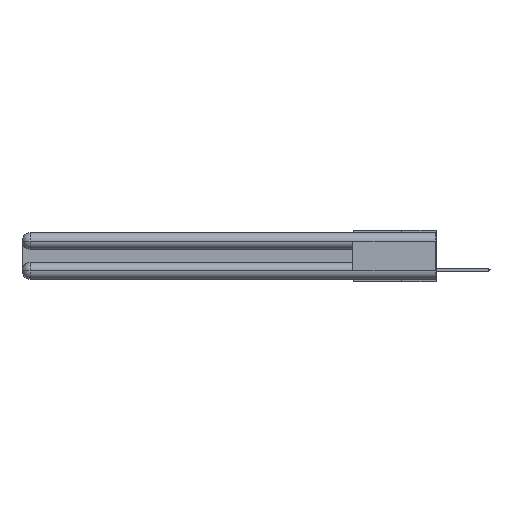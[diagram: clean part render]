
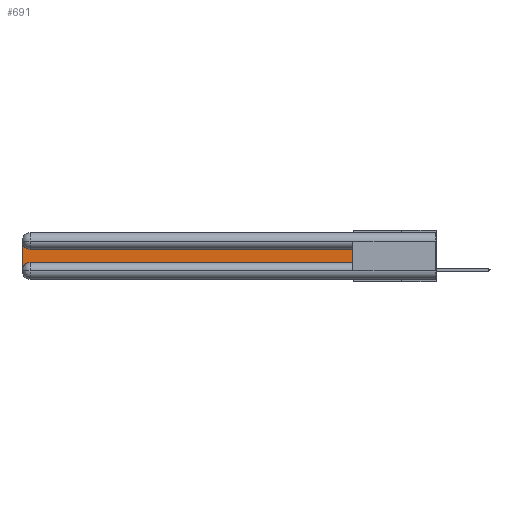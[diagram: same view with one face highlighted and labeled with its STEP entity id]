
A CAD part, left-side view. The second image highlights one B-rep face of the part: STEP entity #691.
In plain terms, the highlighted planar face has unit normal (-1, 0, 0).
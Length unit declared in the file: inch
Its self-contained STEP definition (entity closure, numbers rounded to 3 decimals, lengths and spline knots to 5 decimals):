
#261 = CARTESIAN_POINT ( 'NONE',  ( 0.075, 0.6, -0.2175 ) ) ;
#691 = ADVANCED_FACE ( 'NONE', ( #5377 ), #24101, .F. ) ;
#938 = CARTESIAN_POINT ( 'NONE',  ( 0.075, 0.6, -0.1225 ) ) ;
#1121 = DIRECTION ( 'NONE',  ( 0., 0., 1. ) ) ;
#1133 = CIRCLE ( 'NONE', #24353, 0.06 ) ;
#1188 = DIRECTION ( 'NONE',  ( 1., 0., 0. ) ) ;
#2538 = VERTEX_POINT ( 'NONE', #26113 ) ;
#2850 = DIRECTION ( 'NONE',  ( 1., 0., 0. ) ) ;
#3032 = VECTOR ( 'NONE', #1121, 39.37008 ) ;
#3155 = EDGE_CURVE ( 'NONE', #12133, #13346, #20397, .T. ) ;
#3655 = AXIS2_PLACEMENT_3D ( 'NONE', #5633, #14016, #5889 ) ;
#4423 = AXIS2_PLACEMENT_3D ( 'NONE', #25682, #1188, #17885 ) ;
#4706 = DIRECTION ( 'NONE',  ( 0., 0., -1. ) ) ;
#4826 = CARTESIAN_POINT ( 'NONE',  ( 0.075, 2.94, -0.0625 ) ) ;
#5377 = FACE_OUTER_BOUND ( 'NONE', #7575, .T. ) ;
#5633 = CARTESIAN_POINT ( 'NONE',  ( 0.075, 3., -0.1225 ) ) ;
#5889 = DIRECTION ( 'NONE',  ( 0., 0., -1. ) ) ;
#6248 = VERTEX_POINT ( 'NONE', #18762 ) ;
#6718 = EDGE_CURVE ( 'NONE', #15944, #20426, #1133, .T. ) ;
#7150 = CARTESIAN_POINT ( 'NONE',  ( 0.075, 3., -0.0625 ) ) ;
#7454 = DIRECTION ( 'NONE',  ( 0., 1., 0. ) ) ;
#7575 = EDGE_LOOP ( 'NONE', ( #8621, #14292, #20727, #9318, #16063, #13437 ) ) ;
#8621 = ORIENTED_EDGE ( 'NONE', *, *, #22195, .T. ) ;
#9318 = ORIENTED_EDGE ( 'NONE', *, *, #10266, .T. ) ;
#10266 = EDGE_CURVE ( 'NONE', #2538, #6248, #14144, .T. ) ;
#10718 = CARTESIAN_POINT ( 'NONE',  ( 0.075, 0.6, -0.2175 ) ) ;
#12133 = VERTEX_POINT ( 'NONE', #261 ) ;
#12501 = VECTOR ( 'NONE', #7454, 39.37008 ) ;
#13346 = VERTEX_POINT ( 'NONE', #25940 ) ;
#13437 = ORIENTED_EDGE ( 'NONE', *, *, #3155, .T. ) ;
#14016 = DIRECTION ( 'NONE',  ( 1., 0., 0. ) ) ;
#14144 = CIRCLE ( 'NONE', #4423, 0.06 ) ;
#14153 = LINE ( 'NONE', #10718, #23050 ) ;
#14292 = ORIENTED_EDGE ( 'NONE', *, *, #6718, .T. ) ;
#15944 = VERTEX_POINT ( 'NONE', #26277 ) ;
#16063 = ORIENTED_EDGE ( 'NONE', *, *, #23849, .T. ) ;
#16623 = EDGE_CURVE ( 'NONE', #20426, #2538, #23799, .T. ) ;
#17281 = DIRECTION ( 'NONE',  ( 0., 0., -1. ) ) ;
#17885 = DIRECTION ( 'NONE',  ( 0., 0., -1. ) ) ;
#18422 = VECTOR ( 'NONE', #4706, 39.37008 ) ;
#18762 = CARTESIAN_POINT ( 'NONE',  ( 0.075, 2.94, -0.2175 ) ) ;
#20397 = LINE ( 'NONE', #21815, #3032 ) ;
#20426 = VERTEX_POINT ( 'NONE', #7150 ) ;
#20606 = DIRECTION ( 'NONE',  ( 0., -1., 0. ) ) ;
#20727 = ORIENTED_EDGE ( 'NONE', *, *, #16623, .T. ) ;
#21815 = CARTESIAN_POINT ( 'NONE',  ( 0.075, 0.6, -0.2175 ) ) ;
#22195 = EDGE_CURVE ( 'NONE', #13346, #15944, #24956, .T. ) ;
#23050 = VECTOR ( 'NONE', #20606, 39.37008 ) ;
#23799 = LINE ( 'NONE', #25060, #18422 ) ;
#23849 = EDGE_CURVE ( 'NONE', #6248, #12133, #14153, .T. ) ;
#24101 = PLANE ( 'NONE',  #3655 ) ;
#24353 = AXIS2_PLACEMENT_3D ( 'NONE', #4826, #2850, #17281 ) ;
#24956 = LINE ( 'NONE', #938, #12501 ) ;
#25060 = CARTESIAN_POINT ( 'NONE',  ( 0.075, 3., -0.2175 ) ) ;
#25682 = CARTESIAN_POINT ( 'NONE',  ( 0.075, 2.94, -0.2775 ) ) ;
#25940 = CARTESIAN_POINT ( 'NONE',  ( 0.075, 0.6, -0.1225 ) ) ;
#26113 = CARTESIAN_POINT ( 'NONE',  ( 0.075, 3., -0.2775 ) ) ;
#26277 = CARTESIAN_POINT ( 'NONE',  ( 0.075, 2.94, -0.1225 ) ) ;
